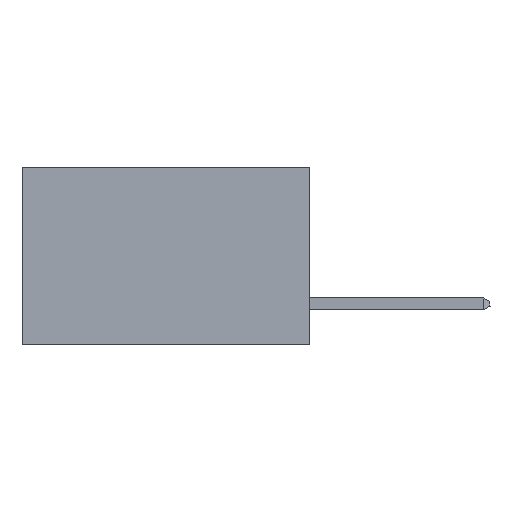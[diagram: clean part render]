
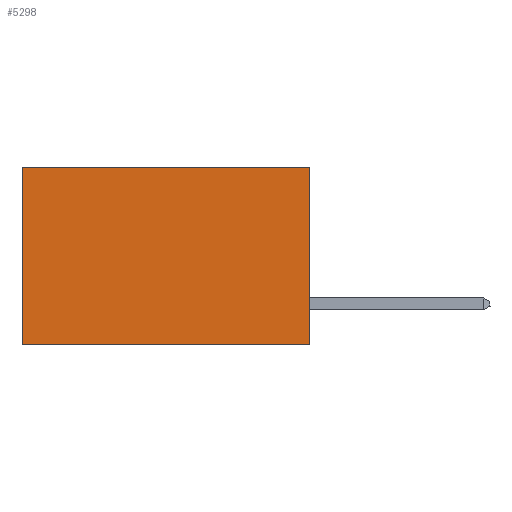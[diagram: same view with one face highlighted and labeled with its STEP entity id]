
A CAD part, left-side view. The second image highlights one B-rep face of the part: STEP entity #5298.
In plain terms, the highlighted planar face has unit normal (-1, 0, 0).
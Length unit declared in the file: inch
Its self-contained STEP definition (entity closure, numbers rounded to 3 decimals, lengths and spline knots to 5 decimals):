
#329 = DIRECTION ( 'NONE',  ( 0., 0., -1. ) ) ;
#615 = CARTESIAN_POINT ( 'NONE',  ( 0.2875, 0., 0. ) ) ;
#641 = CARTESIAN_POINT ( 'NONE',  ( 0.2875, 0., -0.37 ) ) ;
#846 = DIRECTION ( 'NONE',  ( 0., 0., -1. ) ) ;
#3259 = VERTEX_POINT ( 'NONE', #8926 ) ;
#4394 = ORIENTED_EDGE ( 'NONE', *, *, #24149, .T. ) ;
#5298 = ADVANCED_FACE ( 'NONE', ( #8100 ), #6472, .F. ) ;
#6257 = VERTEX_POINT ( 'NONE', #28051 ) ;
#6454 = CARTESIAN_POINT ( 'NONE',  ( 0.2875, 0.6, 0. ) ) ;
#6472 = PLANE ( 'NONE',  #34824 ) ;
#7203 = ORIENTED_EDGE ( 'NONE', *, *, #30610, .T. ) ;
#8100 = FACE_OUTER_BOUND ( 'NONE', #40270, .T. ) ;
#8926 = CARTESIAN_POINT ( 'NONE',  ( 0.2875, 0.6, 0. ) ) ;
#8951 = VERTEX_POINT ( 'NONE', #24278 ) ;
#9662 = DIRECTION ( 'NONE',  ( 1., 0., 0. ) ) ;
#10576 = CARTESIAN_POINT ( 'NONE',  ( 0.2875, 0., 0. ) ) ;
#10994 = DIRECTION ( 'NONE',  ( 0., 0., -1. ) ) ;
#13496 = CARTESIAN_POINT ( 'NONE',  ( 0.2875, 0.6, -0.37 ) ) ;
#16121 = VECTOR ( 'NONE', #29123, 39.37008 ) ;
#17200 = VERTEX_POINT ( 'NONE', #13496 ) ;
#18102 = DIRECTION ( 'NONE',  ( 0., 1., 0. ) ) ;
#18227 = CARTESIAN_POINT ( 'NONE',  ( 0.2875, 0., 0. ) ) ;
#20693 = LINE ( 'NONE', #18227, #39646 ) ;
#22063 = VECTOR ( 'NONE', #846, 39.37008 ) ;
#22467 = LINE ( 'NONE', #6454, #25906 ) ;
#24149 = EDGE_CURVE ( 'NONE', #6257, #3259, #20693, .T. ) ;
#24278 = CARTESIAN_POINT ( 'NONE',  ( 0.2875, 0., -0.37 ) ) ;
#25576 = LINE ( 'NONE', #641, #16121 ) ;
#25906 = VECTOR ( 'NONE', #10994, 39.37008 ) ;
#26066 = LINE ( 'NONE', #10576, #22063 ) ;
#28051 = CARTESIAN_POINT ( 'NONE',  ( 0.2875, 0., 0. ) ) ;
#28717 = EDGE_CURVE ( 'NONE', #8951, #17200, #25576, .T. ) ;
#29123 = DIRECTION ( 'NONE',  ( 0., 1., 0. ) ) ;
#30610 = EDGE_CURVE ( 'NONE', #3259, #17200, #22467, .T. ) ;
#31180 = ORIENTED_EDGE ( 'NONE', *, *, #40646, .F. ) ;
#33486 = ORIENTED_EDGE ( 'NONE', *, *, #28717, .F. ) ;
#34824 = AXIS2_PLACEMENT_3D ( 'NONE', #615, #9662, #329 ) ;
#39646 = VECTOR ( 'NONE', #18102, 39.37008 ) ;
#40270 = EDGE_LOOP ( 'NONE', ( #7203, #33486, #31180, #4394 ) ) ;
#40646 = EDGE_CURVE ( 'NONE', #6257, #8951, #26066, .T. ) ;
